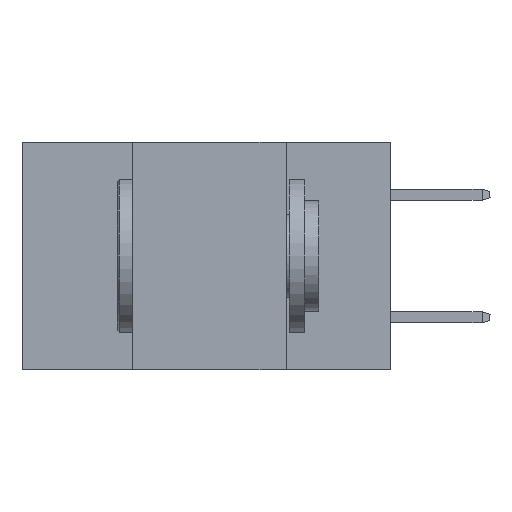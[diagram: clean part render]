
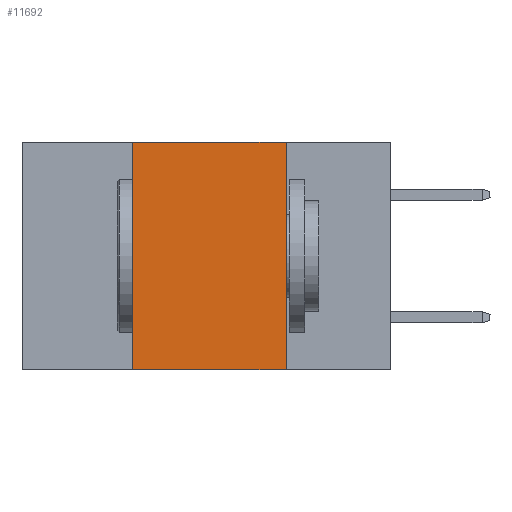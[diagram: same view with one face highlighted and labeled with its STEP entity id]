
A CAD part, left-side view. The second image highlights one B-rep face of the part: STEP entity #11692.
In plain terms, the highlighted planar face has unit normal (-1, 0, 0).
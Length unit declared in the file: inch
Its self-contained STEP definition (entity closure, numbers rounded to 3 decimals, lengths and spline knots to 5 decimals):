
#932 = DIRECTION ( 'NONE',  ( 0., 0., -1. ) ) ;
#1365 = CARTESIAN_POINT ( 'NONE',  ( 0., 0.17, 0. ) ) ;
#1863 = CARTESIAN_POINT ( 'NONE',  ( 0., 0.6, -0.37 ) ) ;
#3231 = ORIENTED_EDGE ( 'NONE', *, *, #42474, .T. ) ;
#4328 = VECTOR ( 'NONE', #34444, 39.37008 ) ;
#5932 = CARTESIAN_POINT ( 'NONE',  ( 0., 0.42, 0. ) ) ;
#8006 = LINE ( 'NONE', #35736, #35193 ) ;
#8235 = ORIENTED_EDGE ( 'NONE', *, *, #30454, .F. ) ;
#9381 = CARTESIAN_POINT ( 'NONE',  ( 0., 0.42, -0.37 ) ) ;
#11198 = VERTEX_POINT ( 'NONE', #9381 ) ;
#11236 = LINE ( 'NONE', #1365, #33421 ) ;
#11692 = ADVANCED_FACE ( 'NONE', ( #18377 ), #37751, .F. ) ;
#11950 = EDGE_CURVE ( 'NONE', #36442, #35705, #8006, .T. ) ;
#12489 = EDGE_LOOP ( 'NONE', ( #8235, #34376, #30793, #3231 ) ) ;
#13312 = DIRECTION ( 'NONE',  ( 1., 0., 0. ) ) ;
#18377 = FACE_OUTER_BOUND ( 'NONE', #12489, .T. ) ;
#19319 = DIRECTION ( 'NONE',  ( 0., -1., 0. ) ) ;
#21723 = LINE ( 'NONE', #44860, #4328 ) ;
#26464 = CARTESIAN_POINT ( 'NONE',  ( 0., 0.17, -0.37 ) ) ;
#26932 = DIRECTION ( 'NONE',  ( 0., 0., -1. ) ) ;
#29808 = CARTESIAN_POINT ( 'NONE',  ( 0., 0.17, 0. ) ) ;
#30454 = EDGE_CURVE ( 'NONE', #35705, #35721, #11236, .T. ) ;
#30793 = ORIENTED_EDGE ( 'NONE', *, *, #43484, .F. ) ;
#31201 = AXIS2_PLACEMENT_3D ( 'NONE', #40900, #13312, #26932 ) ;
#33421 = VECTOR ( 'NONE', #932, 39.37008 ) ;
#33774 = LINE ( 'NONE', #1863, #38133 ) ;
#34376 = ORIENTED_EDGE ( 'NONE', *, *, #11950, .F. ) ;
#34444 = DIRECTION ( 'NONE',  ( 0., 0., 1. ) ) ;
#35193 = VECTOR ( 'NONE', #35452, 39.37008 ) ;
#35452 = DIRECTION ( 'NONE',  ( 0., -1., 0. ) ) ;
#35705 = VERTEX_POINT ( 'NONE', #29808 ) ;
#35721 = VERTEX_POINT ( 'NONE', #26464 ) ;
#35736 = CARTESIAN_POINT ( 'NONE',  ( 0., 0.6, 0. ) ) ;
#36442 = VERTEX_POINT ( 'NONE', #5932 ) ;
#37751 = PLANE ( 'NONE',  #31201 ) ;
#38133 = VECTOR ( 'NONE', #19319, 39.37008 ) ;
#40900 = CARTESIAN_POINT ( 'NONE',  ( 0., 0.6, 0. ) ) ;
#42474 = EDGE_CURVE ( 'NONE', #11198, #35721, #33774, .T. ) ;
#43484 = EDGE_CURVE ( 'NONE', #11198, #36442, #21723, .T. ) ;
#44860 = CARTESIAN_POINT ( 'NONE',  ( 0., 0.42, 0. ) ) ;
